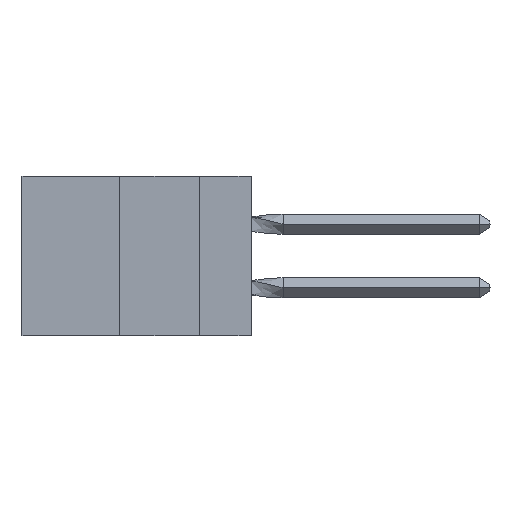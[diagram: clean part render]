
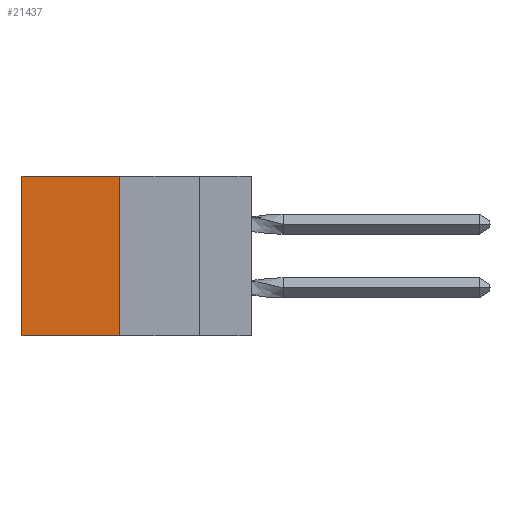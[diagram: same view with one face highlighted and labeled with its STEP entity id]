
A CAD part, left-side view. The second image highlights one B-rep face of the part: STEP entity #21437.
In plain terms, the highlighted planar face has unit normal (-1, 0, 0).
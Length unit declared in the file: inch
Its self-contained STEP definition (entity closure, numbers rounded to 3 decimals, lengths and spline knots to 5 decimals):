
#22 = VERTEX_POINT ( 'NONE', #3673 ) ;
#3673 = CARTESIAN_POINT ( 'NONE',  ( 0.305, 0.72, 0. ) ) ;
#3876 = LINE ( 'NONE', #24335, #16005 ) ;
#4632 = DIRECTION ( 'NONE',  ( 1., 0., 0. ) ) ;
#4649 = VERTEX_POINT ( 'NONE', #13694 ) ;
#5432 = LINE ( 'NONE', #10682, #19980 ) ;
#7104 = VECTOR ( 'NONE', #19134, 39.37008 ) ;
#7775 = FACE_OUTER_BOUND ( 'NONE', #9855, .T. ) ;
#9066 = CARTESIAN_POINT ( 'NONE',  ( 0.305, 0.413, -0.5 ) ) ;
#9371 = VERTEX_POINT ( 'NONE', #14078 ) ;
#9566 = LINE ( 'NONE', #9066, #10142 ) ;
#9855 = EDGE_LOOP ( 'NONE', ( #22800, #16024, #20169, #15414 ) ) ;
#10019 = CARTESIAN_POINT ( 'NONE',  ( 0.305, 0.413, -0.5 ) ) ;
#10142 = VECTOR ( 'NONE', #24210, 39.37008 ) ;
#10682 = CARTESIAN_POINT ( 'NONE',  ( 0.305, 0.413, 0. ) ) ;
#11002 = EDGE_CURVE ( 'NONE', #9371, #19468, #9566, .T. ) ;
#11896 = EDGE_CURVE ( 'NONE', #19468, #4649, #3876, .T. ) ;
#12022 = DIRECTION ( 'NONE',  ( 0., 0., -1. ) ) ;
#12216 = EDGE_CURVE ( 'NONE', #22, #4649, #21946, .T. ) ;
#12944 = DIRECTION ( 'NONE',  ( 0., 1., 0. ) ) ;
#13694 = CARTESIAN_POINT ( 'NONE',  ( 0.305, 0.72, -0.5 ) ) ;
#14078 = CARTESIAN_POINT ( 'NONE',  ( 0.305, 0.413, 0. ) ) ;
#15414 = ORIENTED_EDGE ( 'NONE', *, *, #15923, .T. ) ;
#15817 = PLANE ( 'NONE',  #16159 ) ;
#15923 = EDGE_CURVE ( 'NONE', #9371, #22, #5432, .T. ) ;
#15978 = CARTESIAN_POINT ( 'NONE',  ( 0.305, 0.413, -0.5 ) ) ;
#16005 = VECTOR ( 'NONE', #12944, 39.37008 ) ;
#16024 = ORIENTED_EDGE ( 'NONE', *, *, #11896, .F. ) ;
#16159 = AXIS2_PLACEMENT_3D ( 'NONE', #15978, #4632, #12022 ) ;
#17226 = CARTESIAN_POINT ( 'NONE',  ( 0.305, 0.72, -0.5 ) ) ;
#19134 = DIRECTION ( 'NONE',  ( 0., 0., -1. ) ) ;
#19468 = VERTEX_POINT ( 'NONE', #10019 ) ;
#19980 = VECTOR ( 'NONE', #22183, 39.37008 ) ;
#20169 = ORIENTED_EDGE ( 'NONE', *, *, #11002, .F. ) ;
#21437 = ADVANCED_FACE ( 'NONE', ( #7775 ), #15817, .F. ) ;
#21946 = LINE ( 'NONE', #17226, #7104 ) ;
#22183 = DIRECTION ( 'NONE',  ( 0., 1., 0. ) ) ;
#22800 = ORIENTED_EDGE ( 'NONE', *, *, #12216, .T. ) ;
#24210 = DIRECTION ( 'NONE',  ( 0., 0., -1. ) ) ;
#24335 = CARTESIAN_POINT ( 'NONE',  ( 0.305, 0.413, -0.5 ) ) ;
